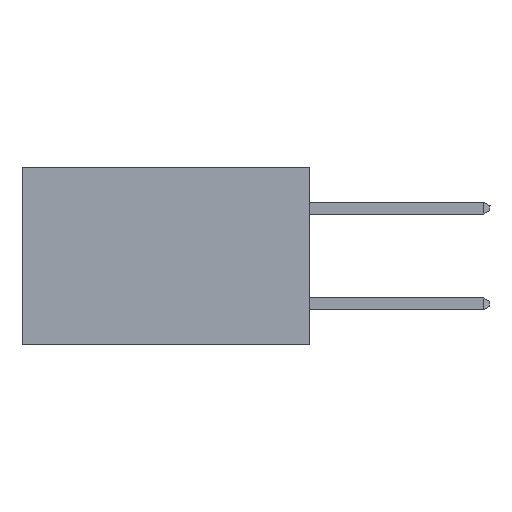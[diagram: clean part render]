
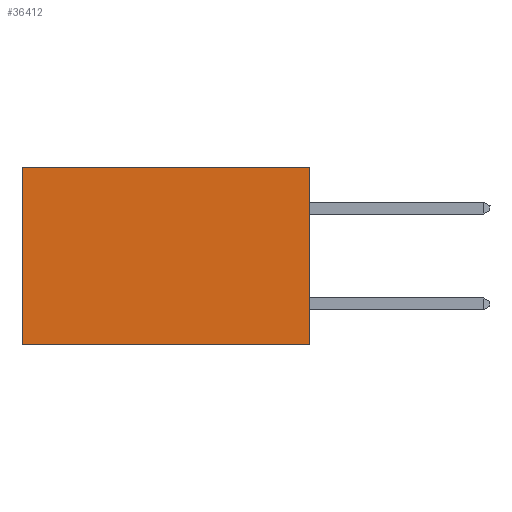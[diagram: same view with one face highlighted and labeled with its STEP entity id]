
A CAD part, left-side view. The second image highlights one B-rep face of the part: STEP entity #36412.
In plain terms, the highlighted planar face has unit normal (-1, 0, 0).
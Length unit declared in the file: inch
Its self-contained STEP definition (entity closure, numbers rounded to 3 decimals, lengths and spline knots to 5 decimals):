
#339 = AXIS2_PLACEMENT_3D ( 'NONE', #1270, #33471, #7225 ) ;
#451 = LINE ( 'NONE', #26198, #23945 ) ;
#1270 = CARTESIAN_POINT ( 'NONE',  ( 0.2875, 0., 0. ) ) ;
#2708 = DIRECTION ( 'NONE',  ( 0., 1., 0. ) ) ;
#2861 = EDGE_CURVE ( 'NONE', #19771, #20523, #451, .T. ) ;
#4173 = FACE_OUTER_BOUND ( 'NONE', #20674, .T. ) ;
#4257 = PLANE ( 'NONE',  #339 ) ;
#7202 = CARTESIAN_POINT ( 'NONE',  ( 0.2875, 0., -0.37 ) ) ;
#7225 = DIRECTION ( 'NONE',  ( 0., 0., -1. ) ) ;
#7676 = ORIENTED_EDGE ( 'NONE', *, *, #26765, .T. ) ;
#9580 = CARTESIAN_POINT ( 'NONE',  ( 0.2875, 0., 0. ) ) ;
#11700 = EDGE_CURVE ( 'NONE', #37737, #21194, #15281, .T. ) ;
#11915 = ORIENTED_EDGE ( 'NONE', *, *, #11700, .T. ) ;
#12511 = DIRECTION ( 'NONE',  ( 0., 1., 0. ) ) ;
#15281 = LINE ( 'NONE', #9580, #35802 ) ;
#15618 = CARTESIAN_POINT ( 'NONE',  ( 0.2875, 0., 0. ) ) ;
#15746 = ORIENTED_EDGE ( 'NONE', *, *, #37643, .F. ) ;
#19387 = CARTESIAN_POINT ( 'NONE',  ( 0.2875, 0.6, 0. ) ) ;
#19771 = VERTEX_POINT ( 'NONE', #7202 ) ;
#20523 = VERTEX_POINT ( 'NONE', #30860 ) ;
#20674 = EDGE_LOOP ( 'NONE', ( #7676, #31206, #15746, #11915 ) ) ;
#21194 = VERTEX_POINT ( 'NONE', #19387 ) ;
#23945 = VECTOR ( 'NONE', #2708, 39.37008 ) ;
#24333 = DIRECTION ( 'NONE',  ( 0., 0., -1. ) ) ;
#24715 = CARTESIAN_POINT ( 'NONE',  ( 0.2875, 0., 0. ) ) ;
#25144 = DIRECTION ( 'NONE',  ( 0., 0., -1. ) ) ;
#25717 = LINE ( 'NONE', #31009, #32545 ) ;
#26198 = CARTESIAN_POINT ( 'NONE',  ( 0.2875, 0., -0.37 ) ) ;
#26765 = EDGE_CURVE ( 'NONE', #21194, #20523, #25717, .T. ) ;
#27075 = LINE ( 'NONE', #15618, #35711 ) ;
#30860 = CARTESIAN_POINT ( 'NONE',  ( 0.2875, 0.6, -0.37 ) ) ;
#31009 = CARTESIAN_POINT ( 'NONE',  ( 0.2875, 0.6, 0. ) ) ;
#31206 = ORIENTED_EDGE ( 'NONE', *, *, #2861, .F. ) ;
#32545 = VECTOR ( 'NONE', #25144, 39.37008 ) ;
#33471 = DIRECTION ( 'NONE',  ( 1., 0., 0. ) ) ;
#35711 = VECTOR ( 'NONE', #24333, 39.37008 ) ;
#35802 = VECTOR ( 'NONE', #12511, 39.37008 ) ;
#36412 = ADVANCED_FACE ( 'NONE', ( #4173 ), #4257, .F. ) ;
#37643 = EDGE_CURVE ( 'NONE', #37737, #19771, #27075, .T. ) ;
#37737 = VERTEX_POINT ( 'NONE', #24715 ) ;
